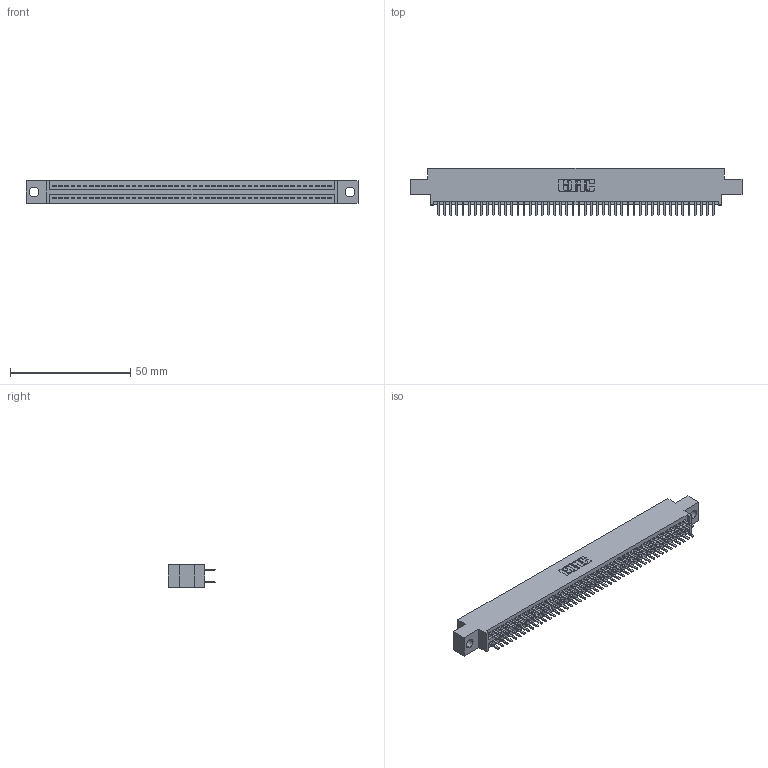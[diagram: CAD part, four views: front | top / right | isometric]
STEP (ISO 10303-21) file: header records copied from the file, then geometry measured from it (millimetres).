
FILE_DESCRIPTION (( 'STEP AP203' ), '1' );
FILE_NAME ('345-092-520-804.STEP', '2018-10-04T20:02:03', ( '' ), ( '' ), 'SwSTEP 2.0', 'SolidWorks 2016', '' );
FILE_SCHEMA (( 'CONFIG_CONTROL_DESIGN' ));
Length unit declared in the file: inch
Products named in the file (3): 345 Part_0.170 Offset - 0.156 Dia-TH; 345-092-520-804; 345-292-001_345-293-120
Assembly tree (93 placements, depth 2):
  345-092-520-804
    345 Part_0.170 Offset - 0.156 Dia-TH
    345-292-001_345-293-120  x92
Bounding box: 138.05 x 19.68 x 9.4 mm (x, y, z)
Volume: 13205.7 mm3; surface area: 19470.3 mm2
Topology: 93 solids, 93 shells, 5098 faces, 14797 edges, 9618 vertices
Faces by surface type: plane 3304, cylinder 1794
Entity records: 35803 total; most frequent: CARTESIAN_POINT 6012, ORIENTED_EDGE 5934, DIRECTION 5283, EDGE_CURVE 2967, VECTOR 2647, LINE 2647, VERTEX_POINT 1974, AXIS2_PLACEMENT_3D 1318
